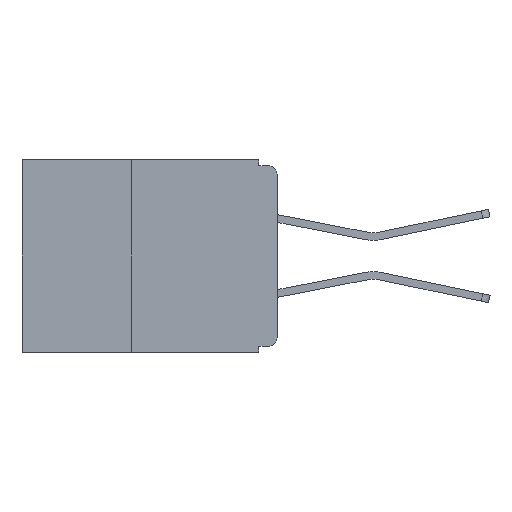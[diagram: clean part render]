
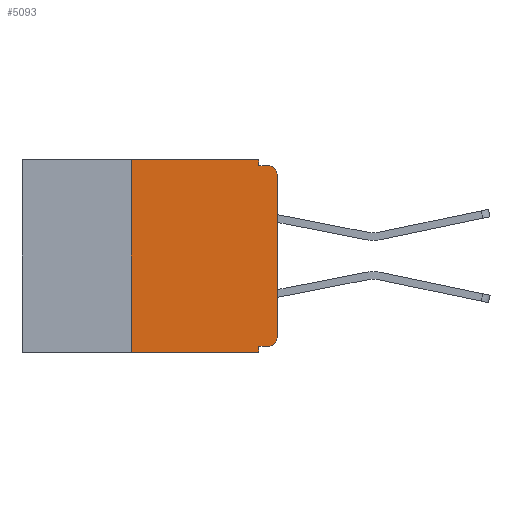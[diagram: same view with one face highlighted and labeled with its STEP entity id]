
A CAD part, left-side view. The second image highlights one B-rep face of the part: STEP entity #5093.
In plain terms, the highlighted planar face has unit normal (-1, 0, 0).
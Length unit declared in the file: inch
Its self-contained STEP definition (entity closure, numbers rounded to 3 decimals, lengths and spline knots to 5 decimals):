
#75 = VECTOR ( 'NONE', #7880, 39.37008 ) ;
#128 = CARTESIAN_POINT ( 'NONE',  ( 0., 0., -0.025 ) ) ;
#604 = DIRECTION ( 'NONE',  ( 0., -1., 0. ) ) ;
#644 = CARTESIAN_POINT ( 'NONE',  ( 0., 0.437, -0.33 ) ) ;
#676 = DIRECTION ( 'NONE',  ( 0., -1., 0. ) ) ;
#713 = ORIENTED_EDGE ( 'NONE', *, *, #6890, .F. ) ;
#747 = DIRECTION ( 'NONE',  ( -1., 0., 0. ) ) ;
#860 = EDGE_CURVE ( 'NONE', #8762, #3928, #1642, .T. ) ;
#1023 = DIRECTION ( 'NONE',  ( 0., 0., 1. ) ) ;
#1355 = CARTESIAN_POINT ( 'NONE',  ( 0., 0., 0. ) ) ;
#1611 = DIRECTION ( 'NONE',  ( 0., 0., -1. ) ) ;
#1624 = CARTESIAN_POINT ( 'NONE',  ( 0., 0., -0.32 ) ) ;
#1631 = ORIENTED_EDGE ( 'NONE', *, *, #1749, .T. ) ;
#1642 = LINE ( 'NONE', #6820, #3563 ) ;
#1744 = AXIS2_PLACEMENT_3D ( 'NONE', #1822, #3582, #8034 ) ;
#1749 = EDGE_CURVE ( 'NONE', #7085, #1761, #4795, .T. ) ;
#1761 = VERTEX_POINT ( 'NONE', #10513 ) ;
#1822 = CARTESIAN_POINT ( 'NONE',  ( 0., 0.437, 0. ) ) ;
#1905 = VECTOR ( 'NONE', #8093, 39.37008 ) ;
#2035 = CARTESIAN_POINT ( 'NONE',  ( 0., 0.031, -0.33 ) ) ;
#2163 = LINE ( 'NONE', #9849, #1905 ) ;
#2168 = CARTESIAN_POINT ( 'NONE',  ( 0., 0.031, -0.32 ) ) ;
#2551 = AXIS2_PLACEMENT_3D ( 'NONE', #9013, #10840, #5455 ) ;
#2616 = ORIENTED_EDGE ( 'NONE', *, *, #4698, .T. ) ;
#2643 = EDGE_LOOP ( 'NONE', ( #5548, #1631, #10743, #8829, #8838, #5751, #8753, #3267, #713, #2616 ) ) ;
#2823 = LINE ( 'NONE', #3236, #10618 ) ;
#3236 = CARTESIAN_POINT ( 'NONE',  ( 0., 0.437, 0. ) ) ;
#3267 = ORIENTED_EDGE ( 'NONE', *, *, #860, .F. ) ;
#3300 = EDGE_CURVE ( 'NONE', #11358, #6813, #4220, .T. ) ;
#3563 = VECTOR ( 'NONE', #8688, 39.37008 ) ;
#3582 = DIRECTION ( 'NONE',  ( 1., 0., 0. ) ) ;
#3613 = CARTESIAN_POINT ( 'NONE',  ( 0., 0.25, -0.33 ) ) ;
#3770 = AXIS2_PLACEMENT_3D ( 'NONE', #9579, #747, #1611 ) ;
#3928 = VERTEX_POINT ( 'NONE', #2035 ) ;
#4220 = LINE ( 'NONE', #3613, #8387 ) ;
#4655 = VERTEX_POINT ( 'NONE', #10407 ) ;
#4698 = EDGE_CURVE ( 'NONE', #4655, #8637, #11553, .T. ) ;
#4756 = CARTESIAN_POINT ( 'NONE',  ( 0., 0.031, 0. ) ) ;
#4795 = CIRCLE ( 'NONE', #3770, 0.015 ) ;
#5093 = ADVANCED_FACE ( 'NONE', ( #7973 ), #8867, .F. ) ;
#5136 = VECTOR ( 'NONE', #9613, 39.37008 ) ;
#5372 = LINE ( 'NONE', #1355, #6608 ) ;
#5444 = LINE ( 'NONE', #644, #10879 ) ;
#5449 = EDGE_CURVE ( 'NONE', #9425, #1761, #7488, .T. ) ;
#5455 = DIRECTION ( 'NONE',  ( 0., 0., -1. ) ) ;
#5548 = ORIENTED_EDGE ( 'NONE', *, *, #7915, .T. ) ;
#5751 = ORIENTED_EDGE ( 'NONE', *, *, #3300, .F. ) ;
#5764 = LINE ( 'NONE', #1624, #75 ) ;
#6579 = EDGE_CURVE ( 'NONE', #10832, #9425, #2163, .T. ) ;
#6608 = VECTOR ( 'NONE', #6671, 39.37008 ) ;
#6671 = DIRECTION ( 'NONE',  ( 0., 0., 1. ) ) ;
#6813 = VERTEX_POINT ( 'NONE', #9533 ) ;
#6820 = CARTESIAN_POINT ( 'NONE',  ( 0., 0.031, -0.33 ) ) ;
#6890 = EDGE_CURVE ( 'NONE', #4655, #8762, #5764, .T. ) ;
#7085 = VERTEX_POINT ( 'NONE', #128 ) ;
#7488 = LINE ( 'NONE', #9538, #5136 ) ;
#7880 = DIRECTION ( 'NONE',  ( 0., 1., 0. ) ) ;
#7915 = EDGE_CURVE ( 'NONE', #8637, #7085, #5372, .T. ) ;
#7973 = FACE_OUTER_BOUND ( 'NONE', #2643, .T. ) ;
#8034 = DIRECTION ( 'NONE',  ( 0., 0., -1. ) ) ;
#8093 = DIRECTION ( 'NONE',  ( 0., 0., -1. ) ) ;
#8387 = VECTOR ( 'NONE', #1023, 39.37008 ) ;
#8587 = CARTESIAN_POINT ( 'NONE',  ( 0., 0.031, -0.01 ) ) ;
#8637 = VERTEX_POINT ( 'NONE', #8965 ) ;
#8688 = DIRECTION ( 'NONE',  ( 0., 0., -1. ) ) ;
#8753 = ORIENTED_EDGE ( 'NONE', *, *, #9934, .T. ) ;
#8762 = VERTEX_POINT ( 'NONE', #2168 ) ;
#8829 = ORIENTED_EDGE ( 'NONE', *, *, #6579, .F. ) ;
#8838 = ORIENTED_EDGE ( 'NONE', *, *, #9437, .F. ) ;
#8867 = PLANE ( 'NONE',  #1744 ) ;
#8965 = CARTESIAN_POINT ( 'NONE',  ( 0., 0., -0.305 ) ) ;
#9013 = CARTESIAN_POINT ( 'NONE',  ( 0., 0.015, -0.305 ) ) ;
#9425 = VERTEX_POINT ( 'NONE', #8587 ) ;
#9437 = EDGE_CURVE ( 'NONE', #6813, #10832, #2823, .T. ) ;
#9460 = CARTESIAN_POINT ( 'NONE',  ( 0., 0.25, -0.33 ) ) ;
#9533 = CARTESIAN_POINT ( 'NONE',  ( 0., 0.25, 0. ) ) ;
#9538 = CARTESIAN_POINT ( 'NONE',  ( 0., 0., -0.01 ) ) ;
#9579 = CARTESIAN_POINT ( 'NONE',  ( 0., 0.015, -0.025 ) ) ;
#9613 = DIRECTION ( 'NONE',  ( 0., -1., 0. ) ) ;
#9849 = CARTESIAN_POINT ( 'NONE',  ( 0., 0.031, 0. ) ) ;
#9934 = EDGE_CURVE ( 'NONE', #11358, #3928, #5444, .T. ) ;
#10407 = CARTESIAN_POINT ( 'NONE',  ( 0., 0.015, -0.32 ) ) ;
#10513 = CARTESIAN_POINT ( 'NONE',  ( 0., 0.015, -0.01 ) ) ;
#10618 = VECTOR ( 'NONE', #676, 39.37008 ) ;
#10743 = ORIENTED_EDGE ( 'NONE', *, *, #5449, .F. ) ;
#10832 = VERTEX_POINT ( 'NONE', #4756 ) ;
#10840 = DIRECTION ( 'NONE',  ( -1., 0., 0. ) ) ;
#10879 = VECTOR ( 'NONE', #604, 39.37008 ) ;
#11358 = VERTEX_POINT ( 'NONE', #9460 ) ;
#11553 = CIRCLE ( 'NONE', #2551, 0.015 ) ;
